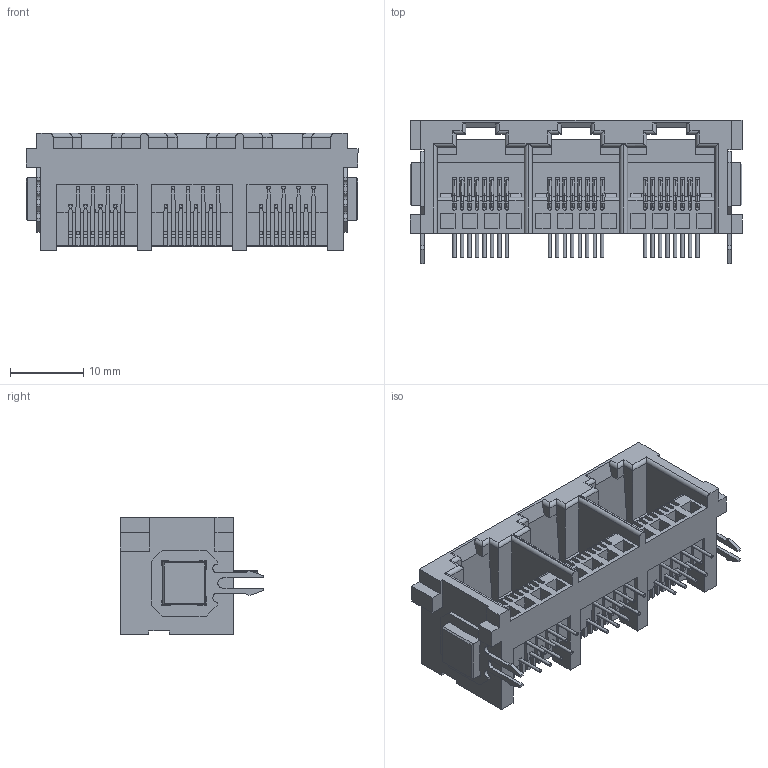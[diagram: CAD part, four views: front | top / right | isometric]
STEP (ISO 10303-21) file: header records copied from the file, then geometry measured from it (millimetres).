
FILE_DESCRIPTION (( 'STEP AP203' ), '1' );
FILE_NAME ('RJG2038832P00013.STEP', '2020-01-20T18:30:16', ( '' ), ( '' ), 'SwSTEP 2.0', 'SolidWorks 2016', '' );
FILE_SCHEMA (( 'CONFIG_CONTROL_DESIGN' ));
Length unit declared in the file: millimetre
Products named in the file (6): G2 Insulator; G2 Contact Lock; RJG2038832P00013; G2 Boardlock2; G2 Contacts; G2 Boardlock1
Assembly tree (9 placements, depth 2):
  RJG2038832P00013
    G2 Insulator
    G2 Boardlock1
    G2 Boardlock2
    G2 Contacts  x3
    G2 Contact Lock  x3
Bounding box: 45.28 x 19.54 x 16 mm (x, y, z)
Volume: 4876.3 mm3; surface area: 9570.8 mm2
Topology: 30 solids, 30 shells, 1835 faces, 5428 edges, 3610 vertices
Faces by surface type: plane 1210, cylinder 457, bspline 168
Entity records: 42785 total; most frequent: CARTESIAN_POINT 11740, ORIENTED_EDGE 6920, DIRECTION 5489, EDGE_CURVE 3460, LINE 2439, VECTOR 2439, VERTEX_POINT 2294, AXIS2_PLACEMENT_3D 1525
